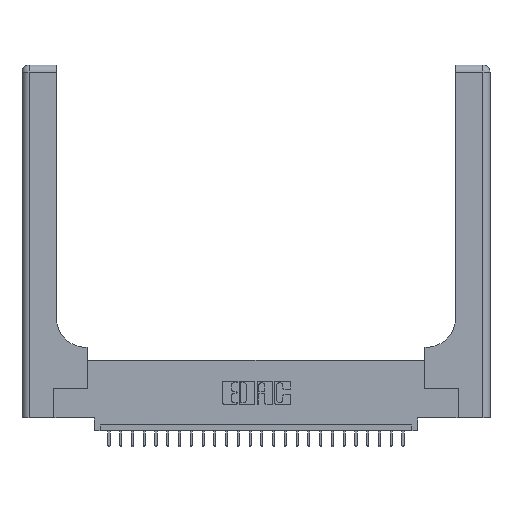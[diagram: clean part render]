
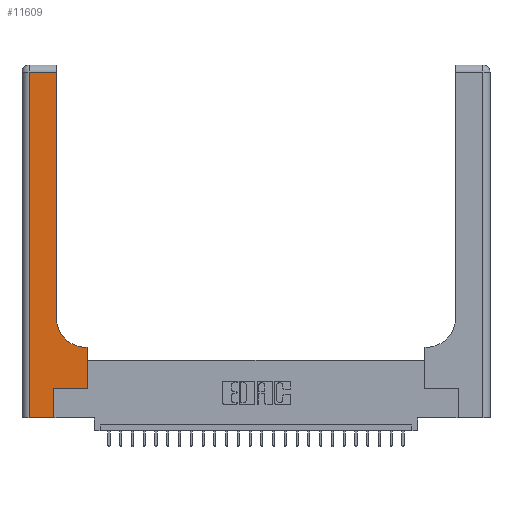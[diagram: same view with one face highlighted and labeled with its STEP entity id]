
A CAD part, top view. The second image highlights one B-rep face of the part: STEP entity #11609.
In plain terms, the highlighted planar face has unit normal (0, 0, 1).
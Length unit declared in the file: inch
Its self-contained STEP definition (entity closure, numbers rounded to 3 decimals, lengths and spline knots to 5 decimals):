
#33 = DIRECTION ( 'NONE',  ( 0., 0., -1. ) ) ;
#426 = ORIENTED_EDGE ( 'NONE', *, *, #26418, .T. ) ;
#1101 = CARTESIAN_POINT ( 'NONE',  ( 0.269, 0.25, 0.37 ) ) ;
#1513 = DIRECTION ( 'NONE',  ( 0., 1., 0. ) ) ;
#1738 = ORIENTED_EDGE ( 'NONE', *, *, #6926, .T. ) ;
#1976 = VECTOR ( 'NONE', #4550, 39.37008 ) ;
#3063 = EDGE_CURVE ( 'NONE', #16514, #17209, #9554, .T. ) ;
#3856 = VECTOR ( 'NONE', #4725, 39.37008 ) ;
#3911 = AXIS2_PLACEMENT_3D ( 'NONE', #19874, #13744, #7574 ) ;
#4372 = EDGE_CURVE ( 'NONE', #8396, #5652, #15411, .T. ) ;
#4550 = DIRECTION ( 'NONE',  ( -1., 0., 0. ) ) ;
#4725 = DIRECTION ( 'NONE',  ( 1., 0., 0. ) ) ;
#5381 = EDGE_CURVE ( 'NONE', #25830, #8396, #12967, .T. ) ;
#5551 = ORIENTED_EDGE ( 'NONE', *, *, #15425, .T. ) ;
#5652 = VERTEX_POINT ( 'NONE', #1101 ) ;
#5983 = AXIS2_PLACEMENT_3D ( 'NONE', #8723, #33, #12821 ) ;
#6534 = PLANE ( 'NONE',  #5983 ) ;
#6590 = DIRECTION ( 'NONE',  ( 0., -1., 0. ) ) ;
#6926 = EDGE_CURVE ( 'NONE', #5652, #19093, #25430, .T. ) ;
#6938 = DIRECTION ( 'NONE',  ( 0., 1., 0. ) ) ;
#7027 = CARTESIAN_POINT ( 'NONE',  ( 0.5585, 0.25, 0.37 ) ) ;
#7449 = ORIENTED_EDGE ( 'NONE', *, *, #17537, .T. ) ;
#7574 = DIRECTION ( 'NONE',  ( 1., 0., 0. ) ) ;
#8029 = EDGE_CURVE ( 'NONE', #13794, #25830, #10703, .T. ) ;
#8396 = VERTEX_POINT ( 'NONE', #12351 ) ;
#8475 = CARTESIAN_POINT ( 'NONE',  ( 0.5415, 0.6, 0.37 ) ) ;
#8723 = CARTESIAN_POINT ( 'NONE',  ( 0., 3., 0.37 ) ) ;
#8997 = LINE ( 'NONE', #17328, #23623 ) ;
#9554 = LINE ( 'NONE', #26388, #22204 ) ;
#10703 = LINE ( 'NONE', #19017, #24642 ) ;
#11145 = VECTOR ( 'NONE', #25683, 39.37008 ) ;
#11294 = CARTESIAN_POINT ( 'NONE',  ( 0.269, 0., 0.37 ) ) ;
#11481 = DIRECTION ( 'NONE',  ( 0., 1., 0. ) ) ;
#11609 = ADVANCED_FACE ( 'NONE', ( #25253 ), #6534, .F. ) ;
#11971 = VERTEX_POINT ( 'NONE', #8475 ) ;
#12351 = CARTESIAN_POINT ( 'NONE',  ( 0.269, 0., 0.37 ) ) ;
#12821 = DIRECTION ( 'NONE',  ( -1., 0., 0. ) ) ;
#12967 = LINE ( 'NONE', #26096, #3856 ) ;
#13208 = CARTESIAN_POINT ( 'NONE',  ( 0.2915, 0.6, 0.37 ) ) ;
#13257 = LINE ( 'NONE', #13387, #26196 ) ;
#13387 = CARTESIAN_POINT ( 'NONE',  ( 0., 2.94, 0.37 ) ) ;
#13744 = DIRECTION ( 'NONE',  ( 0., 0., -1. ) ) ;
#13794 = VERTEX_POINT ( 'NONE', #26084 ) ;
#15275 = ORIENTED_EDGE ( 'NONE', *, *, #4372, .T. ) ;
#15411 = LINE ( 'NONE', #11294, #16116 ) ;
#15425 = EDGE_CURVE ( 'NONE', #17209, #13794, #13257, .T. ) ;
#16116 = VECTOR ( 'NONE', #1513, 39.37008 ) ;
#16126 = EDGE_LOOP ( 'NONE', ( #17812, #5551, #20302, #24055, #15275, #1738, #426, #17006, #7449 ) ) ;
#16514 = VERTEX_POINT ( 'NONE', #26524 ) ;
#17006 = ORIENTED_EDGE ( 'NONE', *, *, #21794, .T. ) ;
#17209 = VERTEX_POINT ( 'NONE', #23043 ) ;
#17221 = CARTESIAN_POINT ( 'NONE',  ( 0.269, 0.25, 0.37 ) ) ;
#17303 = LINE ( 'NONE', #13208, #1976 ) ;
#17328 = CARTESIAN_POINT ( 'NONE',  ( 0.5585, 0.25, 0.37 ) ) ;
#17537 = EDGE_CURVE ( 'NONE', #11971, #16514, #20574, .T. ) ;
#17812 = ORIENTED_EDGE ( 'NONE', *, *, #3063, .T. ) ;
#19017 = CARTESIAN_POINT ( 'NONE',  ( 0.06, 3., 0.37 ) ) ;
#19093 = VERTEX_POINT ( 'NONE', #7027 ) ;
#19401 = DIRECTION ( 'NONE',  ( -1., 0., 0. ) ) ;
#19874 = CARTESIAN_POINT ( 'NONE',  ( 0.5415, 0.85, 0.37 ) ) ;
#20302 = ORIENTED_EDGE ( 'NONE', *, *, #8029, .T. ) ;
#20574 = CIRCLE ( 'NONE', #3911, 0.25 ) ;
#21794 = EDGE_CURVE ( 'NONE', #26225, #11971, #17303, .T. ) ;
#22131 = CARTESIAN_POINT ( 'NONE',  ( 0.06, 0., 0.37 ) ) ;
#22204 = VECTOR ( 'NONE', #11481, 39.37008 ) ;
#23043 = CARTESIAN_POINT ( 'NONE',  ( 0.2915, 2.94, 0.37 ) ) ;
#23623 = VECTOR ( 'NONE', #6938, 39.37008 ) ;
#24055 = ORIENTED_EDGE ( 'NONE', *, *, #5381, .T. ) ;
#24642 = VECTOR ( 'NONE', #6590, 39.37008 ) ;
#25253 = FACE_OUTER_BOUND ( 'NONE', #16126, .T. ) ;
#25430 = LINE ( 'NONE', #17221, #11145 ) ;
#25683 = DIRECTION ( 'NONE',  ( 1., 0., 0. ) ) ;
#25830 = VERTEX_POINT ( 'NONE', #22131 ) ;
#26084 = CARTESIAN_POINT ( 'NONE',  ( 0.06, 2.94, 0.37 ) ) ;
#26096 = CARTESIAN_POINT ( 'NONE',  ( 0., 0., 0.37 ) ) ;
#26196 = VECTOR ( 'NONE', #19401, 39.37008 ) ;
#26225 = VERTEX_POINT ( 'NONE', #26939 ) ;
#26388 = CARTESIAN_POINT ( 'NONE',  ( 0.2915, 3., 0.37 ) ) ;
#26418 = EDGE_CURVE ( 'NONE', #19093, #26225, #8997, .T. ) ;
#26524 = CARTESIAN_POINT ( 'NONE',  ( 0.2915, 0.85, 0.37 ) ) ;
#26939 = CARTESIAN_POINT ( 'NONE',  ( 0.5585, 0.6, 0.37 ) ) ;
